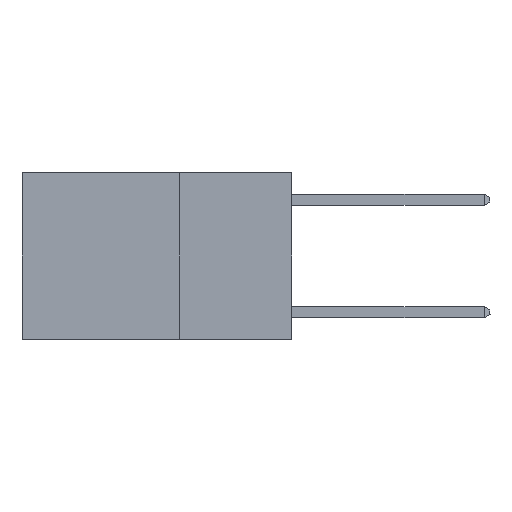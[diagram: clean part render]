
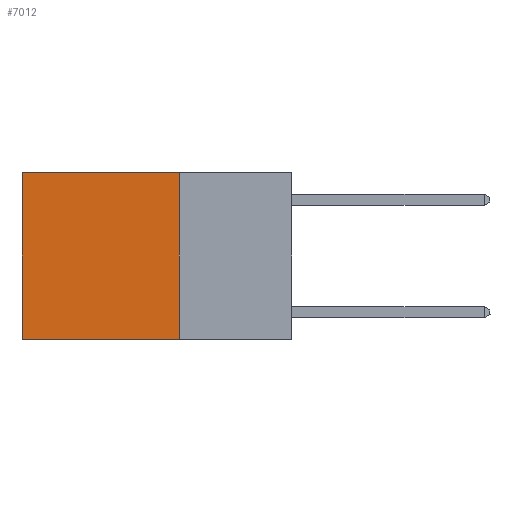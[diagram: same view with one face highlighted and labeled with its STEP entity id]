
A CAD part, left-side view. The second image highlights one B-rep face of the part: STEP entity #7012.
In plain terms, the highlighted planar face has unit normal (-1, 0, 0).
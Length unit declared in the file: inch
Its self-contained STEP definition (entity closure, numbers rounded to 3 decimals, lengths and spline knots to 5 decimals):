
#319 = DIRECTION ( 'NONE',  ( 0., 1., 0. ) ) ;
#326 = VECTOR ( 'NONE', #8990, 39.37008 ) ;
#345 = CARTESIAN_POINT ( 'NONE',  ( 0.2625, 0.25, 0. ) ) ;
#695 = AXIS2_PLACEMENT_3D ( 'NONE', #9532, #10477, #4556 ) ;
#775 = CARTESIAN_POINT ( 'NONE',  ( 0.2625, 0.6, 0. ) ) ;
#943 = LINE ( 'NONE', #1485, #11212 ) ;
#1485 = CARTESIAN_POINT ( 'NONE',  ( 0.2625, 0.25, 0. ) ) ;
#1776 = CARTESIAN_POINT ( 'NONE',  ( 0.2625, 0.6, 0. ) ) ;
#2536 = EDGE_LOOP ( 'NONE', ( #5071, #7257, #5881, #9324 ) ) ;
#3036 = VERTEX_POINT ( 'NONE', #9116 ) ;
#3238 = VERTEX_POINT ( 'NONE', #345 ) ;
#3353 = CARTESIAN_POINT ( 'NONE',  ( 0.2625, 0.25, -0.37 ) ) ;
#4339 = CARTESIAN_POINT ( 'NONE',  ( 0.2625, 0.6, -0.37 ) ) ;
#4395 = EDGE_CURVE ( 'NONE', #3036, #4994, #10451, .T. ) ;
#4556 = DIRECTION ( 'NONE',  ( 0., 0., -1. ) ) ;
#4628 = VERTEX_POINT ( 'NONE', #1776 ) ;
#4994 = VERTEX_POINT ( 'NONE', #4339 ) ;
#5071 = ORIENTED_EDGE ( 'NONE', *, *, #11616, .T. ) ;
#5878 = LINE ( 'NONE', #775, #8207 ) ;
#5881 = ORIENTED_EDGE ( 'NONE', *, *, #8574, .F. ) ;
#7012 = ADVANCED_FACE ( 'NONE', ( #11879 ), #8537, .F. ) ;
#7257 = ORIENTED_EDGE ( 'NONE', *, *, #4395, .F. ) ;
#7853 = VECTOR ( 'NONE', #319, 39.37008 ) ;
#8207 = VECTOR ( 'NONE', #11741, 39.37008 ) ;
#8537 = PLANE ( 'NONE',  #695 ) ;
#8574 = EDGE_CURVE ( 'NONE', #3238, #3036, #10937, .T. ) ;
#8990 = DIRECTION ( 'NONE',  ( 0., 0., -1. ) ) ;
#9037 = CARTESIAN_POINT ( 'NONE',  ( 0.2625, 0.25, 0. ) ) ;
#9116 = CARTESIAN_POINT ( 'NONE',  ( 0.2625, 0.25, -0.37 ) ) ;
#9324 = ORIENTED_EDGE ( 'NONE', *, *, #12643, .T. ) ;
#9532 = CARTESIAN_POINT ( 'NONE',  ( 0.2625, 0.25, 0. ) ) ;
#10451 = LINE ( 'NONE', #3353, #7853 ) ;
#10458 = DIRECTION ( 'NONE',  ( 0., 1., 0. ) ) ;
#10477 = DIRECTION ( 'NONE',  ( 1., 0., 0. ) ) ;
#10937 = LINE ( 'NONE', #9037, #326 ) ;
#11212 = VECTOR ( 'NONE', #10458, 39.37008 ) ;
#11616 = EDGE_CURVE ( 'NONE', #4628, #4994, #5878, .T. ) ;
#11741 = DIRECTION ( 'NONE',  ( 0., 0., -1. ) ) ;
#11879 = FACE_OUTER_BOUND ( 'NONE', #2536, .T. ) ;
#12643 = EDGE_CURVE ( 'NONE', #3238, #4628, #943, .T. ) ;
